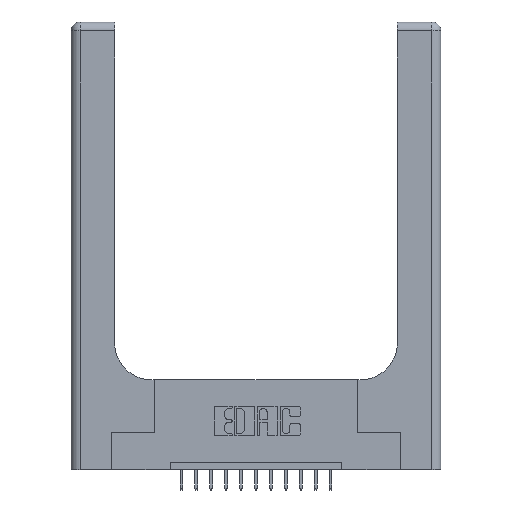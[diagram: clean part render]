
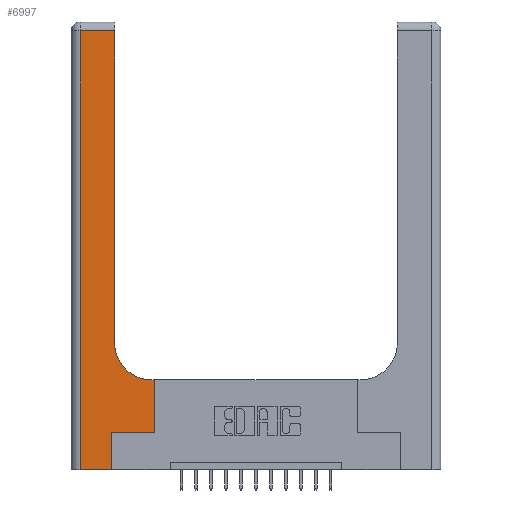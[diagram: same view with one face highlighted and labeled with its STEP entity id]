
A CAD part, top view. The second image highlights one B-rep face of the part: STEP entity #6997.
In plain terms, the highlighted planar face has unit normal (0, 0, 1).
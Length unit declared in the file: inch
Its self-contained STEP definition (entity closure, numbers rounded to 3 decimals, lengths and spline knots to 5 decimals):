
#251 = CARTESIAN_POINT ( 'NONE',  ( 0.5585, 0.25, 0.37 ) ) ;
#284 = VECTOR ( 'NONE', #12442, 39.37008 ) ;
#978 = CARTESIAN_POINT ( 'NONE',  ( 0.2915, 0.6, 0.37 ) ) ;
#1272 = DIRECTION ( 'NONE',  ( 1., 0., 0. ) ) ;
#1696 = EDGE_CURVE ( 'NONE', #6669, #10040, #17145, .T. ) ;
#1917 = CARTESIAN_POINT ( 'NONE',  ( 0., 2.94, 0.37 ) ) ;
#2024 = ORIENTED_EDGE ( 'NONE', *, *, #10124, .T. ) ;
#2100 = DIRECTION ( 'NONE',  ( -1., 0., 0. ) ) ;
#2604 = CARTESIAN_POINT ( 'NONE',  ( 0.5415, 0.85, 0.37 ) ) ;
#2682 = EDGE_CURVE ( 'NONE', #14802, #10650, #10334, .T. ) ;
#3016 = DIRECTION ( 'NONE',  ( 0., 0., -1. ) ) ;
#3174 = ORIENTED_EDGE ( 'NONE', *, *, #3898, .T. ) ;
#3264 = DIRECTION ( 'NONE',  ( 0., 1., 0. ) ) ;
#3429 = CARTESIAN_POINT ( 'NONE',  ( 0.2915, 3., 0.37 ) ) ;
#3898 = EDGE_CURVE ( 'NONE', #10650, #10706, #16902, .T. ) ;
#4859 = CARTESIAN_POINT ( 'NONE',  ( 0.269, 0.25, 0.37 ) ) ;
#4973 = LINE ( 'NONE', #10473, #284 ) ;
#5027 = EDGE_CURVE ( 'NONE', #10706, #12806, #14249, .T. ) ;
#5180 = VERTEX_POINT ( 'NONE', #12175 ) ;
#5218 = CARTESIAN_POINT ( 'NONE',  ( 0.269, 0.25, 0.37 ) ) ;
#5347 = EDGE_LOOP ( 'NONE', ( #3174, #5931, #14984, #14821, #16538, #15005, #2024, #13656, #14099 ) ) ;
#5695 = DIRECTION ( 'NONE',  ( 0., 1., 0. ) ) ;
#5709 = CARTESIAN_POINT ( 'NONE',  ( 0., 3., 0.37 ) ) ;
#5931 = ORIENTED_EDGE ( 'NONE', *, *, #5027, .T. ) ;
#6669 = VERTEX_POINT ( 'NONE', #5218 ) ;
#6943 = VECTOR ( 'NONE', #2100, 39.37008 ) ;
#6997 = ADVANCED_FACE ( 'NONE', ( #9786 ), #10861, .F. ) ;
#7041 = LINE ( 'NONE', #251, #15340 ) ;
#7114 = EDGE_CURVE ( 'NONE', #14911, #14802, #13289, .T. ) ;
#7252 = CARTESIAN_POINT ( 'NONE',  ( 0., 0., 0.37 ) ) ;
#7258 = CARTESIAN_POINT ( 'NONE',  ( 0.06, 0., 0.37 ) ) ;
#7747 = CARTESIAN_POINT ( 'NONE',  ( 0.06, 3., 0.37 ) ) ;
#7995 = VERTEX_POINT ( 'NONE', #7258 ) ;
#8017 = DIRECTION ( 'NONE',  ( 0., -1., 0. ) ) ;
#8100 = DIRECTION ( 'NONE',  ( 0., 0., -1. ) ) ;
#8377 = CARTESIAN_POINT ( 'NONE',  ( 0.5585, 0.6, 0.37 ) ) ;
#8405 = VECTOR ( 'NONE', #10359, 39.37008 ) ;
#8418 = CARTESIAN_POINT ( 'NONE',  ( 0.5585, 0.25, 0.37 ) ) ;
#8751 = EDGE_CURVE ( 'NONE', #5180, #6669, #4973, .T. ) ;
#9323 = DIRECTION ( 'NONE',  ( -1., 0., 0. ) ) ;
#9474 = AXIS2_PLACEMENT_3D ( 'NONE', #2604, #8100, #1272 ) ;
#9786 = FACE_OUTER_BOUND ( 'NONE', #5347, .T. ) ;
#10040 = VERTEX_POINT ( 'NONE', #8418 ) ;
#10062 = LINE ( 'NONE', #7252, #11740 ) ;
#10098 = VECTOR ( 'NONE', #3264, 39.37008 ) ;
#10124 = EDGE_CURVE ( 'NONE', #10040, #14911, #7041, .T. ) ;
#10155 = DIRECTION ( 'NONE',  ( 1., 0., 0. ) ) ;
#10334 = CIRCLE ( 'NONE', #9474, 0.25 ) ;
#10359 = DIRECTION ( 'NONE',  ( 1., 0., 0. ) ) ;
#10473 = CARTESIAN_POINT ( 'NONE',  ( 0.269, 0., 0.37 ) ) ;
#10646 = AXIS2_PLACEMENT_3D ( 'NONE', #5709, #3016, #11043 ) ;
#10650 = VERTEX_POINT ( 'NONE', #12051 ) ;
#10660 = VECTOR ( 'NONE', #9323, 39.37008 ) ;
#10706 = VERTEX_POINT ( 'NONE', #11134 ) ;
#10861 = PLANE ( 'NONE',  #10646 ) ;
#11043 = DIRECTION ( 'NONE',  ( -1., 0., 0. ) ) ;
#11134 = CARTESIAN_POINT ( 'NONE',  ( 0.2915, 2.94, 0.37 ) ) ;
#11496 = CARTESIAN_POINT ( 'NONE',  ( 0.06, 2.94, 0.37 ) ) ;
#11713 = VECTOR ( 'NONE', #8017, 39.37008 ) ;
#11740 = VECTOR ( 'NONE', #10155, 39.37008 ) ;
#11808 = LINE ( 'NONE', #7747, #11713 ) ;
#11989 = CARTESIAN_POINT ( 'NONE',  ( 0.5415, 0.6, 0.37 ) ) ;
#12051 = CARTESIAN_POINT ( 'NONE',  ( 0.2915, 0.85, 0.37 ) ) ;
#12175 = CARTESIAN_POINT ( 'NONE',  ( 0.269, 0., 0.37 ) ) ;
#12442 = DIRECTION ( 'NONE',  ( 0., 1., 0. ) ) ;
#12806 = VERTEX_POINT ( 'NONE', #11496 ) ;
#13289 = LINE ( 'NONE', #978, #10660 ) ;
#13656 = ORIENTED_EDGE ( 'NONE', *, *, #7114, .T. ) ;
#14099 = ORIENTED_EDGE ( 'NONE', *, *, #2682, .T. ) ;
#14249 = LINE ( 'NONE', #1917, #6943 ) ;
#14725 = EDGE_CURVE ( 'NONE', #12806, #7995, #11808, .T. ) ;
#14802 = VERTEX_POINT ( 'NONE', #11989 ) ;
#14821 = ORIENTED_EDGE ( 'NONE', *, *, #15849, .T. ) ;
#14911 = VERTEX_POINT ( 'NONE', #8377 ) ;
#14984 = ORIENTED_EDGE ( 'NONE', *, *, #14725, .T. ) ;
#15005 = ORIENTED_EDGE ( 'NONE', *, *, #1696, .T. ) ;
#15340 = VECTOR ( 'NONE', #5695, 39.37008 ) ;
#15849 = EDGE_CURVE ( 'NONE', #7995, #5180, #10062, .T. ) ;
#16538 = ORIENTED_EDGE ( 'NONE', *, *, #8751, .T. ) ;
#16902 = LINE ( 'NONE', #3429, #10098 ) ;
#17145 = LINE ( 'NONE', #4859, #8405 ) ;
